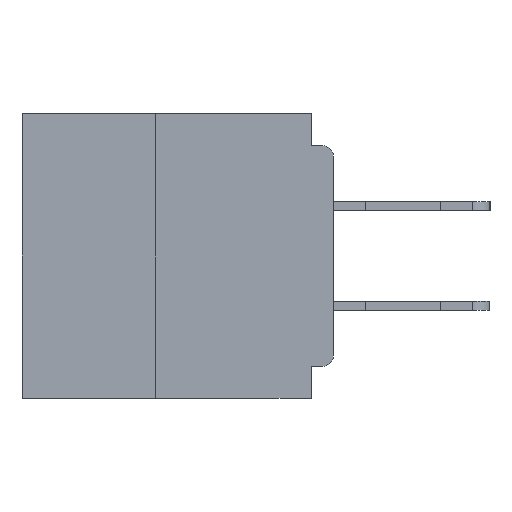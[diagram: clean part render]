
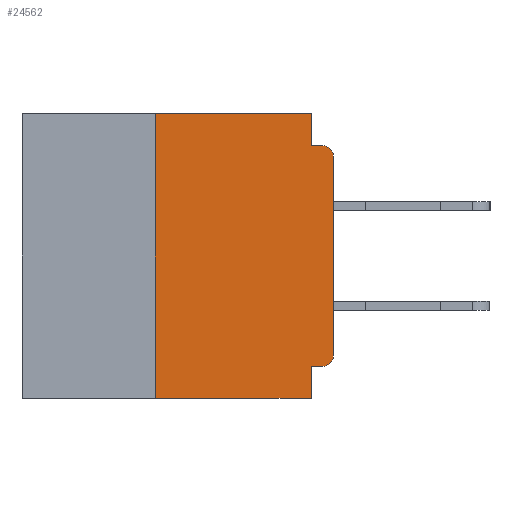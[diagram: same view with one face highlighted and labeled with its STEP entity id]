
A CAD part, left-side view. The second image highlights one B-rep face of the part: STEP entity #24562.
In plain terms, the highlighted planar face has unit normal (-1, 0, 0).
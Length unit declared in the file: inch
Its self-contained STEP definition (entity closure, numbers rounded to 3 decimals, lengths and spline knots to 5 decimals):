
#516 = CARTESIAN_POINT ( 'NONE',  ( 0., 0., -0.34 ) ) ;
#2500 = CIRCLE ( 'NONE', #37959, 0.015 ) ;
#2832 = LINE ( 'NONE', #33673, #26257 ) ;
#2974 = VERTEX_POINT ( 'NONE', #28635 ) ;
#3332 = VERTEX_POINT ( 'NONE', #21542 ) ;
#4737 = ORIENTED_EDGE ( 'NONE', *, *, #26450, .F. ) ;
#6469 = EDGE_CURVE ( 'NONE', #23922, #14358, #22293, .T. ) ;
#7314 = VERTEX_POINT ( 'NONE', #14847 ) ;
#7610 = CARTESIAN_POINT ( 'NONE',  ( 0., 0.437, 0. ) ) ;
#7714 = DIRECTION ( 'NONE',  ( 0., -1., 0. ) ) ;
#8252 = VECTOR ( 'NONE', #16444, 39.37008 ) ;
#9427 = EDGE_CURVE ( 'NONE', #36160, #14407, #24508, .T. ) ;
#9782 = CARTESIAN_POINT ( 'NONE',  ( 0., 0.031, -0.4 ) ) ;
#9965 = CARTESIAN_POINT ( 'NONE',  ( 0., 0.015, -0.355 ) ) ;
#10569 = CARTESIAN_POINT ( 'NONE',  ( 0., 0., 0. ) ) ;
#10852 = DIRECTION ( 'NONE',  ( 1., 0., 0. ) ) ;
#11192 = DIRECTION ( 'NONE',  ( 0., 0., 1. ) ) ;
#11274 = VERTEX_POINT ( 'NONE', #38031 ) ;
#11857 = AXIS2_PLACEMENT_3D ( 'NONE', #7610, #10852, #33087 ) ;
#12327 = DIRECTION ( 'NONE',  ( 0., -1., 0. ) ) ;
#12570 = EDGE_CURVE ( 'NONE', #28791, #2974, #17783, .T. ) ;
#12816 = EDGE_CURVE ( 'NONE', #36160, #20151, #17251, .T. ) ;
#12918 = LINE ( 'NONE', #40795, #37256 ) ;
#13745 = ORIENTED_EDGE ( 'NONE', *, *, #9427, .F. ) ;
#14184 = ORIENTED_EDGE ( 'NONE', *, *, #12570, .F. ) ;
#14358 = VERTEX_POINT ( 'NONE', #18121 ) ;
#14407 = VERTEX_POINT ( 'NONE', #37257 ) ;
#14636 = ORIENTED_EDGE ( 'NONE', *, *, #39935, .T. ) ;
#14847 = CARTESIAN_POINT ( 'NONE',  ( 0., 0.031, 0. ) ) ;
#14992 = CIRCLE ( 'NONE', #25762, 0.015 ) ;
#16444 = DIRECTION ( 'NONE',  ( 0., 1., 0. ) ) ;
#16558 = CARTESIAN_POINT ( 'NONE',  ( 0., 0.015, -0.34 ) ) ;
#17251 = LINE ( 'NONE', #17520, #23700 ) ;
#17442 = LINE ( 'NONE', #37252, #34303 ) ;
#17520 = CARTESIAN_POINT ( 'NONE',  ( 0., 0.437, -0.4 ) ) ;
#17696 = CARTESIAN_POINT ( 'NONE',  ( 0., 0.015, -0.06 ) ) ;
#17783 = LINE ( 'NONE', #29061, #8252 ) ;
#18121 = CARTESIAN_POINT ( 'NONE',  ( 0., 0., -0.06 ) ) ;
#18254 = DIRECTION ( 'NONE',  ( 0., 0., -1. ) ) ;
#19087 = ORIENTED_EDGE ( 'NONE', *, *, #20369, .F. ) ;
#19766 = DIRECTION ( 'NONE',  ( 0., 0., -1. ) ) ;
#20067 = DIRECTION ( 'NONE',  ( 0., 0., 1. ) ) ;
#20151 = VERTEX_POINT ( 'NONE', #9782 ) ;
#20369 = EDGE_CURVE ( 'NONE', #2974, #20151, #2832, .T. ) ;
#20881 = DIRECTION ( 'NONE',  ( 0., 0., -1. ) ) ;
#21542 = CARTESIAN_POINT ( 'NONE',  ( 0., 0.015, -0.045 ) ) ;
#22293 = LINE ( 'NONE', #10569, #28729 ) ;
#22879 = ORIENTED_EDGE ( 'NONE', *, *, #40792, .F. ) ;
#23700 = VECTOR ( 'NONE', #39696, 39.37008 ) ;
#23854 = LINE ( 'NONE', #33059, #39729 ) ;
#23922 = VERTEX_POINT ( 'NONE', #516 ) ;
#24508 = LINE ( 'NONE', #27047, #40373 ) ;
#24562 = ADVANCED_FACE ( 'NONE', ( #33983 ), #26704, .F. ) ;
#24874 = ORIENTED_EDGE ( 'NONE', *, *, #6469, .T. ) ;
#25762 = AXIS2_PLACEMENT_3D ( 'NONE', #17696, #39863, #20881 ) ;
#26257 = VECTOR ( 'NONE', #27304, 39.37008 ) ;
#26450 = EDGE_CURVE ( 'NONE', #7314, #11274, #17442, .T. ) ;
#26704 = PLANE ( 'NONE',  #11857 ) ;
#26844 = EDGE_CURVE ( 'NONE', #14407, #7314, #23854, .T. ) ;
#27047 = CARTESIAN_POINT ( 'NONE',  ( 0., 0.25, -0.4 ) ) ;
#27304 = DIRECTION ( 'NONE',  ( 0., 0., -1. ) ) ;
#28635 = CARTESIAN_POINT ( 'NONE',  ( 0., 0.031, -0.355 ) ) ;
#28640 = CARTESIAN_POINT ( 'NONE',  ( 0., 0.25, -0.4 ) ) ;
#28729 = VECTOR ( 'NONE', #20067, 39.37008 ) ;
#28791 = VERTEX_POINT ( 'NONE', #9965 ) ;
#29061 = CARTESIAN_POINT ( 'NONE',  ( 0., 0., -0.355 ) ) ;
#31707 = ORIENTED_EDGE ( 'NONE', *, *, #26844, .F. ) ;
#33009 = ORIENTED_EDGE ( 'NONE', *, *, #12816, .T. ) ;
#33059 = CARTESIAN_POINT ( 'NONE',  ( 0., 0.437, 0. ) ) ;
#33087 = DIRECTION ( 'NONE',  ( 0., 0., -1. ) ) ;
#33673 = CARTESIAN_POINT ( 'NONE',  ( 0., 0.031, -0.4 ) ) ;
#33983 = FACE_OUTER_BOUND ( 'NONE', #35130, .T. ) ;
#34303 = VECTOR ( 'NONE', #18254, 39.37008 ) ;
#35130 = EDGE_LOOP ( 'NONE', ( #24874, #14636, #22879, #4737, #31707, #13745, #33009, #19087, #14184, #39825 ) ) ;
#36160 = VERTEX_POINT ( 'NONE', #28640 ) ;
#37252 = CARTESIAN_POINT ( 'NONE',  ( 0., 0.031, 0. ) ) ;
#37256 = VECTOR ( 'NONE', #12327, 39.37008 ) ;
#37257 = CARTESIAN_POINT ( 'NONE',  ( 0., 0.25, 0. ) ) ;
#37959 = AXIS2_PLACEMENT_3D ( 'NONE', #16558, #38733, #19766 ) ;
#38031 = CARTESIAN_POINT ( 'NONE',  ( 0., 0.031, -0.045 ) ) ;
#38733 = DIRECTION ( 'NONE',  ( -1., 0., 0. ) ) ;
#39485 = EDGE_CURVE ( 'NONE', #28791, #23922, #2500, .T. ) ;
#39696 = DIRECTION ( 'NONE',  ( 0., -1., 0. ) ) ;
#39729 = VECTOR ( 'NONE', #7714, 39.37008 ) ;
#39825 = ORIENTED_EDGE ( 'NONE', *, *, #39485, .T. ) ;
#39863 = DIRECTION ( 'NONE',  ( -1., 0., 0. ) ) ;
#39935 = EDGE_CURVE ( 'NONE', #14358, #3332, #14992, .T. ) ;
#40373 = VECTOR ( 'NONE', #11192, 39.37008 ) ;
#40792 = EDGE_CURVE ( 'NONE', #11274, #3332, #12918, .T. ) ;
#40795 = CARTESIAN_POINT ( 'NONE',  ( 0., 0., -0.045 ) ) ;
